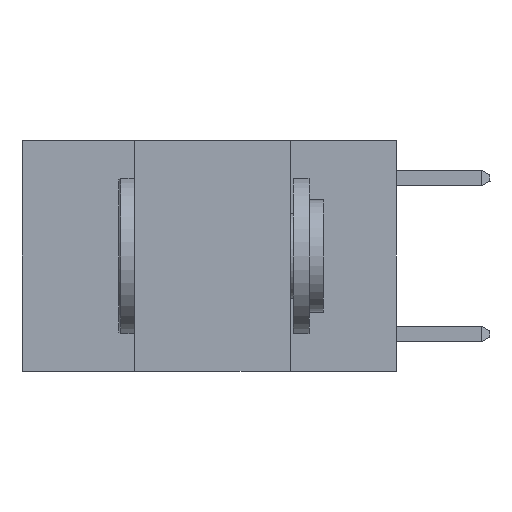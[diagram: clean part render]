
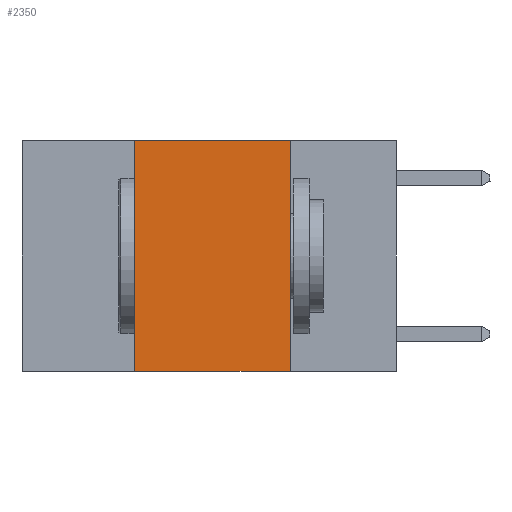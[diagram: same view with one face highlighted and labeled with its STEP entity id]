
A CAD part, left-side view. The second image highlights one B-rep face of the part: STEP entity #2350.
In plain terms, the highlighted planar face has unit normal (-1, 0, 0).
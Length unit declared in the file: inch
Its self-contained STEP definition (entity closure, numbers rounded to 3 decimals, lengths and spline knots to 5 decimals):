
#700 = ORIENTED_EDGE ( 'NONE', *, *, #19221, .F. ) ;
#1131 = CARTESIAN_POINT ( 'NONE',  ( 0., 0.42, 0. ) ) ;
#1527 = DIRECTION ( 'NONE',  ( 0., -1., 0. ) ) ;
#1726 = FACE_OUTER_BOUND ( 'NONE', #5674, .T. ) ;
#2350 = ADVANCED_FACE ( 'NONE', ( #1726 ), #3699, .F. ) ;
#2991 = LINE ( 'NONE', #18704, #13796 ) ;
#3348 = VECTOR ( 'NONE', #20379, 39.37008 ) ;
#3699 = PLANE ( 'NONE',  #15610 ) ;
#5674 = EDGE_LOOP ( 'NONE', ( #19247, #9899, #700, #11051 ) ) ;
#5726 = DIRECTION ( 'NONE',  ( 1., 0., 0. ) ) ;
#6760 = CARTESIAN_POINT ( 'NONE',  ( 0., 0.17, 0. ) ) ;
#6855 = VERTEX_POINT ( 'NONE', #11097 ) ;
#7415 = CARTESIAN_POINT ( 'NONE',  ( 0., 0.42, 0. ) ) ;
#8551 = LINE ( 'NONE', #11027, #3348 ) ;
#9899 = ORIENTED_EDGE ( 'NONE', *, *, #12157, .F. ) ;
#11027 = CARTESIAN_POINT ( 'NONE',  ( 0., 0.17, 0. ) ) ;
#11051 = ORIENTED_EDGE ( 'NONE', *, *, #24224, .T. ) ;
#11097 = CARTESIAN_POINT ( 'NONE',  ( 0., 0.17, -0.37 ) ) ;
#12157 = EDGE_CURVE ( 'NONE', #15547, #18446, #2991, .T. ) ;
#12545 = VECTOR ( 'NONE', #24172, 39.37008 ) ;
#13008 = CARTESIAN_POINT ( 'NONE',  ( 0., 0.6, -0.37 ) ) ;
#13796 = VECTOR ( 'NONE', #1527, 39.37008 ) ;
#14937 = DIRECTION ( 'NONE',  ( 0., 0., 1. ) ) ;
#15098 = CARTESIAN_POINT ( 'NONE',  ( 0., 0.6, 0. ) ) ;
#15219 = VECTOR ( 'NONE', #14937, 39.37008 ) ;
#15547 = VERTEX_POINT ( 'NONE', #1131 ) ;
#15610 = AXIS2_PLACEMENT_3D ( 'NONE', #15098, #5726, #18846 ) ;
#17979 = EDGE_CURVE ( 'NONE', #18446, #6855, #8551, .T. ) ;
#18446 = VERTEX_POINT ( 'NONE', #6760 ) ;
#18704 = CARTESIAN_POINT ( 'NONE',  ( 0., 0.6, 0. ) ) ;
#18846 = DIRECTION ( 'NONE',  ( 0., 0., -1. ) ) ;
#19221 = EDGE_CURVE ( 'NONE', #19747, #15547, #20799, .T. ) ;
#19247 = ORIENTED_EDGE ( 'NONE', *, *, #17979, .F. ) ;
#19747 = VERTEX_POINT ( 'NONE', #21965 ) ;
#20379 = DIRECTION ( 'NONE',  ( 0., 0., -1. ) ) ;
#20799 = LINE ( 'NONE', #7415, #15219 ) ;
#21942 = LINE ( 'NONE', #13008, #12545 ) ;
#21965 = CARTESIAN_POINT ( 'NONE',  ( 0., 0.42, -0.37 ) ) ;
#24172 = DIRECTION ( 'NONE',  ( 0., -1., 0. ) ) ;
#24224 = EDGE_CURVE ( 'NONE', #19747, #6855, #21942, .T. ) ;
